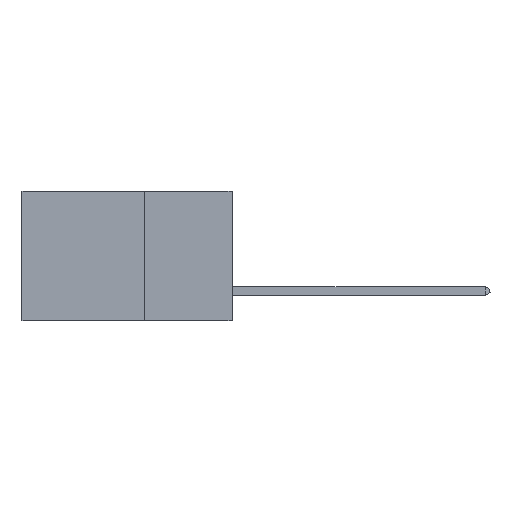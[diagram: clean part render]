
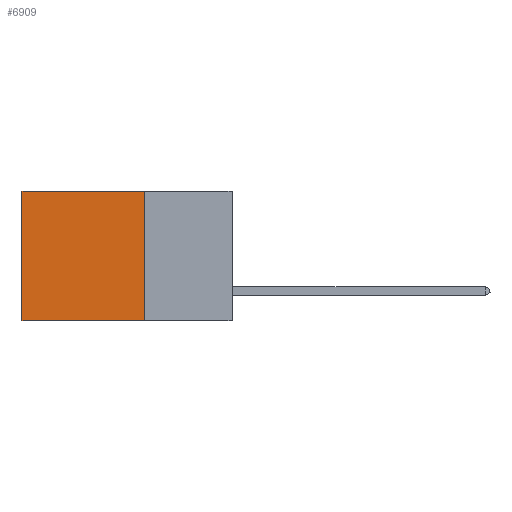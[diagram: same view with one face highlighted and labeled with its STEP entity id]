
A CAD part, left-side view. The second image highlights one B-rep face of the part: STEP entity #6909.
In plain terms, the highlighted planar face has unit normal (-1, 0, 0).
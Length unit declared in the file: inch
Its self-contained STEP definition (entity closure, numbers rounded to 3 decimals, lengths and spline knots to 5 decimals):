
#588 = VECTOR ( 'NONE', #13486, 39.37008 ) ;
#1612 = ORIENTED_EDGE ( 'NONE', *, *, #18359, .T. ) ;
#2133 = LINE ( 'NONE', #3387, #23256 ) ;
#2169 = ORIENTED_EDGE ( 'NONE', *, *, #4948, .F. ) ;
#2170 = EDGE_LOOP ( 'NONE', ( #1612, #5866, #2169, #15975 ) ) ;
#2774 = PLANE ( 'NONE',  #22958 ) ;
#3387 = CARTESIAN_POINT ( 'NONE',  ( 0.2875, 0.25, -0.37 ) ) ;
#4637 = VERTEX_POINT ( 'NONE', #6661 ) ;
#4948 = EDGE_CURVE ( 'NONE', #5777, #4637, #19130, .T. ) ;
#5343 = VERTEX_POINT ( 'NONE', #22961 ) ;
#5777 = VERTEX_POINT ( 'NONE', #20537 ) ;
#5866 = ORIENTED_EDGE ( 'NONE', *, *, #22356, .F. ) ;
#6241 = DIRECTION ( 'NONE',  ( 1., 0., 0. ) ) ;
#6661 = CARTESIAN_POINT ( 'NONE',  ( 0.2875, 0.25, -0.37 ) ) ;
#6770 = DIRECTION ( 'NONE',  ( 0., 1., 0. ) ) ;
#6909 = ADVANCED_FACE ( 'NONE', ( #20267 ), #2774, .F. ) ;
#10759 = DIRECTION ( 'NONE',  ( 0., 0., -1. ) ) ;
#12709 = CARTESIAN_POINT ( 'NONE',  ( 0.2875, 0.25, 0. ) ) ;
#12913 = LINE ( 'NONE', #13894, #14312 ) ;
#13486 = DIRECTION ( 'NONE',  ( 0., 0., -1. ) ) ;
#13894 = CARTESIAN_POINT ( 'NONE',  ( 0.2875, 0.25, 0. ) ) ;
#14051 = DIRECTION ( 'NONE',  ( 0., 1., 0. ) ) ;
#14312 = VECTOR ( 'NONE', #14051, 39.37008 ) ;
#15392 = EDGE_CURVE ( 'NONE', #5777, #5343, #12913, .T. ) ;
#15975 = ORIENTED_EDGE ( 'NONE', *, *, #15392, .T. ) ;
#16243 = VECTOR ( 'NONE', #10759, 39.37008 ) ;
#17091 = VERTEX_POINT ( 'NONE', #19686 ) ;
#17547 = CARTESIAN_POINT ( 'NONE',  ( 0.2875, 0.6, 0. ) ) ;
#18359 = EDGE_CURVE ( 'NONE', #5343, #17091, #19094, .T. ) ;
#19094 = LINE ( 'NONE', #17547, #588 ) ;
#19130 = LINE ( 'NONE', #12709, #16243 ) ;
#19686 = CARTESIAN_POINT ( 'NONE',  ( 0.2875, 0.6, -0.37 ) ) ;
#20267 = FACE_OUTER_BOUND ( 'NONE', #2170, .T. ) ;
#20537 = CARTESIAN_POINT ( 'NONE',  ( 0.2875, 0.25, 0. ) ) ;
#22356 = EDGE_CURVE ( 'NONE', #4637, #17091, #2133, .T. ) ;
#22782 = DIRECTION ( 'NONE',  ( 0., 0., -1. ) ) ;
#22868 = CARTESIAN_POINT ( 'NONE',  ( 0.2875, 0.25, 0. ) ) ;
#22958 = AXIS2_PLACEMENT_3D ( 'NONE', #22868, #6241, #22782 ) ;
#22961 = CARTESIAN_POINT ( 'NONE',  ( 0.2875, 0.6, 0. ) ) ;
#23256 = VECTOR ( 'NONE', #6770, 39.37008 ) ;
